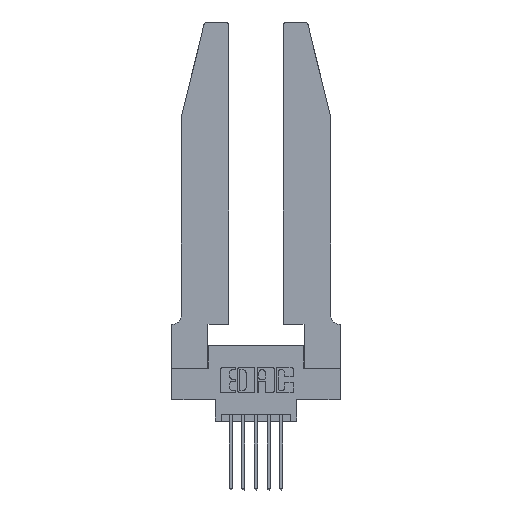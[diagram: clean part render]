
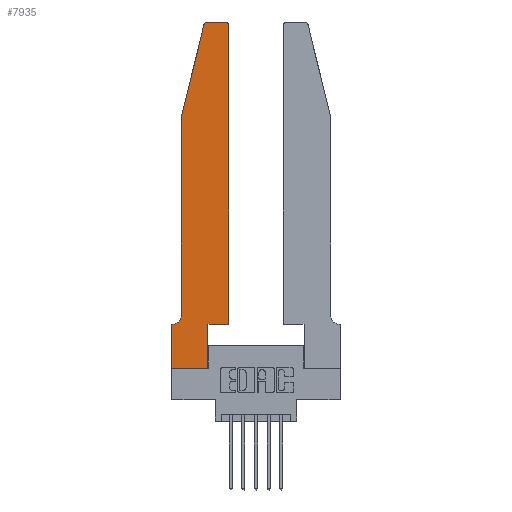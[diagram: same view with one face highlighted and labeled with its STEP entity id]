
A CAD part, top view. The second image highlights one B-rep face of the part: STEP entity #7935.
In plain terms, the highlighted planar face has unit normal (0, 0, 1).
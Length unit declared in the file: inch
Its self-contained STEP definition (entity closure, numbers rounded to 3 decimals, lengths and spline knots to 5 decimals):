
#161 = FACE_OUTER_BOUND ( 'NONE', #5826, .T. ) ;
#242 = CARTESIAN_POINT ( 'NONE',  ( 0.0055, 0.35, 0.37 ) ) ;
#491 = LINE ( 'NONE', #11004, #11185 ) ;
#516 = AXIS2_PLACEMENT_3D ( 'NONE', #3416, #3409, #3398 ) ;
#773 = EDGE_CURVE ( 'NONE', #1426, #12442, #11396, .T. ) ;
#774 = CARTESIAN_POINT ( 'NONE',  ( 0.0755, 2., 0.37 ) ) ;
#805 = ORIENTED_EDGE ( 'NONE', *, *, #7349, .T. ) ;
#967 = LINE ( 'NONE', #3314, #11972 ) ;
#1360 = ORIENTED_EDGE ( 'NONE', *, *, #11991, .T. ) ;
#1403 = ORIENTED_EDGE ( 'NONE', *, *, #7287, .T. ) ;
#1426 = VERTEX_POINT ( 'NONE', #9782 ) ;
#1453 = AXIS2_PLACEMENT_3D ( 'NONE', #6363, #13782, #7434 ) ;
#1861 = CARTESIAN_POINT ( 'NONE',  ( 0.0755, 0.42, 0.37 ) ) ;
#1888 = DIRECTION ( 'NONE',  ( -0.239, -0.971, 0. ) ) ;
#1931 = CARTESIAN_POINT ( 'NONE',  ( 0.284, 2.75, 0.37 ) ) ;
#1974 = ORIENTED_EDGE ( 'NONE', *, *, #3076, .T. ) ;
#2332 = DIRECTION ( 'NONE',  ( 1., 0., 0. ) ) ;
#2338 = DIRECTION ( 'NONE',  ( 0., 0., 1. ) ) ;
#2376 = CARTESIAN_POINT ( 'NONE',  ( 0.284, 2.72, 0.37 ) ) ;
#2385 = CARTESIAN_POINT ( 'NONE',  ( 0.4205, 2.75, 0.37 ) ) ;
#2582 = VERTEX_POINT ( 'NONE', #2385 ) ;
#2764 = ORIENTED_EDGE ( 'NONE', *, *, #7511, .T. ) ;
#2806 = DIRECTION ( 'NONE',  ( -1., 0., 0. ) ) ;
#2833 = VERTEX_POINT ( 'NONE', #1861 ) ;
#2837 = DIRECTION ( 'NONE',  ( 0., 0., -1. ) ) ;
#2844 = DIRECTION ( 'NONE',  ( 0., -1., 0. ) ) ;
#2849 = CARTESIAN_POINT ( 'NONE',  ( 0.0055, 0.42, 0.37 ) ) ;
#2932 = VECTOR ( 'NONE', #10843, 39.37008 ) ;
#3076 = EDGE_CURVE ( 'NONE', #3856, #12609, #11357, .T. ) ;
#3122 = CARTESIAN_POINT ( 'NONE',  ( 0.2865, 0., 0.37 ) ) ;
#3248 = PLANE ( 'NONE',  #1453 ) ;
#3314 = CARTESIAN_POINT ( 'NONE',  ( 0., 0., 0.37 ) ) ;
#3320 = ORIENTED_EDGE ( 'NONE', *, *, #11016, .T. ) ;
#3398 = DIRECTION ( 'NONE',  ( 1., 0., 0. ) ) ;
#3409 = DIRECTION ( 'NONE',  ( 0., 0., 1. ) ) ;
#3416 = CARTESIAN_POINT ( 'NONE',  ( 0.4205, 2.72, 0.37 ) ) ;
#3568 = CARTESIAN_POINT ( 'NONE',  ( 0.2865, 0.35, 0.37 ) ) ;
#3693 = CARTESIAN_POINT ( 'NONE',  ( 0., 0., 0.37 ) ) ;
#3801 = ORIENTED_EDGE ( 'NONE', *, *, #7426, .T. ) ;
#3856 = VERTEX_POINT ( 'NONE', #5271 ) ;
#3857 = CARTESIAN_POINT ( 'NONE',  ( 0.0755, 0.35, 0.37 ) ) ;
#4000 = DIRECTION ( 'NONE',  ( -1., 0., 0. ) ) ;
#4140 = CIRCLE ( 'NONE', #516, 0.03 ) ;
#4176 = AXIS2_PLACEMENT_3D ( 'NONE', #2849, #2837, #2806 ) ;
#4490 = VERTEX_POINT ( 'NONE', #774 ) ;
#4795 = DIRECTION ( 'NONE',  ( 0., -1., 0. ) ) ;
#4877 = AXIS2_PLACEMENT_3D ( 'NONE', #2376, #2338, #2332 ) ;
#4934 = DIRECTION ( 'NONE',  ( 1., 0., 0. ) ) ;
#4971 = CARTESIAN_POINT ( 'NONE',  ( 0.4505, 0.35, 0.37 ) ) ;
#5169 = ORIENTED_EDGE ( 'NONE', *, *, #7148, .T. ) ;
#5271 = CARTESIAN_POINT ( 'NONE',  ( 0.4505, 0.35, 0.37 ) ) ;
#5646 = EDGE_CURVE ( 'NONE', #2582, #10167, #7785, .T. ) ;
#5764 = VECTOR ( 'NONE', #2844, 39.37008 ) ;
#5826 = EDGE_LOOP ( 'NONE', ( #6225, #2764, #1360, #12399, #3801, #1403, #12414, #3320, #12081, #5169, #1974, #805 ) ) ;
#6061 = DIRECTION ( 'NONE',  ( -1., 0., 0. ) ) ;
#6104 = VECTOR ( 'NONE', #4934, 39.37008 ) ;
#6225 = ORIENTED_EDGE ( 'NONE', *, *, #5646, .T. ) ;
#6363 = CARTESIAN_POINT ( 'NONE',  ( 0., 0.35, 0.37 ) ) ;
#6558 = CARTESIAN_POINT ( 'NONE',  ( 0.2605, 2.75, 0.37 ) ) ;
#6582 = VERTEX_POINT ( 'NONE', #8255 ) ;
#6915 = LINE ( 'NONE', #3857, #9752 ) ;
#7132 = VECTOR ( 'NONE', #1888, 39.37008 ) ;
#7148 = EDGE_CURVE ( 'NONE', #9923, #3856, #11413, .T. ) ;
#7236 = CARTESIAN_POINT ( 'NONE',  ( 0.4505, 0.35, 0.37 ) ) ;
#7287 = EDGE_CURVE ( 'NONE', #11195, #1426, #6915, .T. ) ;
#7349 = EDGE_CURVE ( 'NONE', #12609, #2582, #4140, .T. ) ;
#7426 = EDGE_CURVE ( 'NONE', #2833, #11195, #8391, .T. ) ;
#7434 = DIRECTION ( 'NONE',  ( 1., 0., 0. ) ) ;
#7511 = EDGE_CURVE ( 'NONE', #10167, #6582, #10247, .T. ) ;
#7785 = LINE ( 'NONE', #6558, #13107 ) ;
#7935 = ADVANCED_FACE ( 'NONE', ( #161 ), #3248, .T. ) ;
#8164 = CARTESIAN_POINT ( 'NONE',  ( 0.4505, 2.72, 0.37 ) ) ;
#8206 = LINE ( 'NONE', #11117, #10722 ) ;
#8246 = EDGE_CURVE ( 'NONE', #4490, #2833, #8206, .T. ) ;
#8255 = CARTESIAN_POINT ( 'NONE',  ( 0.25487, 2.72718, 0.37 ) ) ;
#8391 = CIRCLE ( 'NONE', #4176, 0.07 ) ;
#9404 = EDGE_CURVE ( 'NONE', #11443, #9923, #491, .T. ) ;
#9617 = DIRECTION ( 'NONE',  ( 1., 0., 0. ) ) ;
#9752 = VECTOR ( 'NONE', #4000, 39.37008 ) ;
#9782 = CARTESIAN_POINT ( 'NONE',  ( 0., 0.35, 0.37 ) ) ;
#9923 = VERTEX_POINT ( 'NONE', #3568 ) ;
#9982 = LINE ( 'NONE', #13508, #7132 ) ;
#10167 = VERTEX_POINT ( 'NONE', #1931 ) ;
#10247 = CIRCLE ( 'NONE', #4877, 0.03 ) ;
#10722 = VECTOR ( 'NONE', #4795, 39.37008 ) ;
#10843 = DIRECTION ( 'NONE',  ( 0., 1., 0. ) ) ;
#11004 = CARTESIAN_POINT ( 'NONE',  ( 0.2865, 0.35, 0.37 ) ) ;
#11016 = EDGE_CURVE ( 'NONE', #12442, #11443, #967, .T. ) ;
#11117 = CARTESIAN_POINT ( 'NONE',  ( 0.0755, 2., 0.37 ) ) ;
#11185 = VECTOR ( 'NONE', #13129, 39.37008 ) ;
#11195 = VERTEX_POINT ( 'NONE', #242 ) ;
#11357 = LINE ( 'NONE', #7236, #2932 ) ;
#11396 = LINE ( 'NONE', #13190, #5764 ) ;
#11413 = LINE ( 'NONE', #4971, #6104 ) ;
#11443 = VERTEX_POINT ( 'NONE', #3122 ) ;
#11972 = VECTOR ( 'NONE', #9617, 39.37008 ) ;
#11991 = EDGE_CURVE ( 'NONE', #6582, #4490, #9982, .T. ) ;
#12081 = ORIENTED_EDGE ( 'NONE', *, *, #9404, .T. ) ;
#12399 = ORIENTED_EDGE ( 'NONE', *, *, #8246, .T. ) ;
#12414 = ORIENTED_EDGE ( 'NONE', *, *, #773, .T. ) ;
#12442 = VERTEX_POINT ( 'NONE', #3693 ) ;
#12609 = VERTEX_POINT ( 'NONE', #8164 ) ;
#13107 = VECTOR ( 'NONE', #6061, 39.37008 ) ;
#13129 = DIRECTION ( 'NONE',  ( 0., 1., 0. ) ) ;
#13190 = CARTESIAN_POINT ( 'NONE',  ( 0., 0., 0.37 ) ) ;
#13508 = CARTESIAN_POINT ( 'NONE',  ( 0.0755, 2., 0.37 ) ) ;
#13782 = DIRECTION ( 'NONE',  ( 0., 0., 1. ) ) ;
